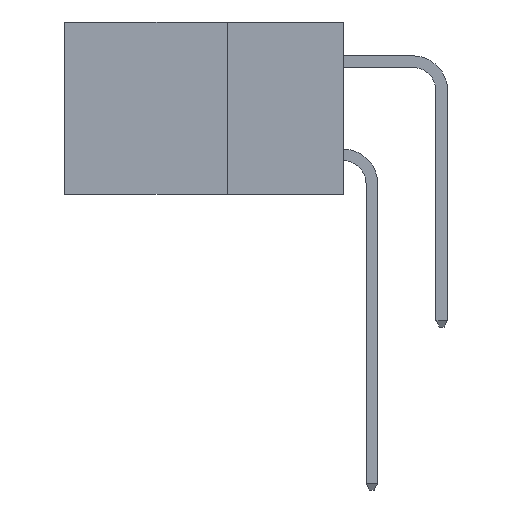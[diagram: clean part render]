
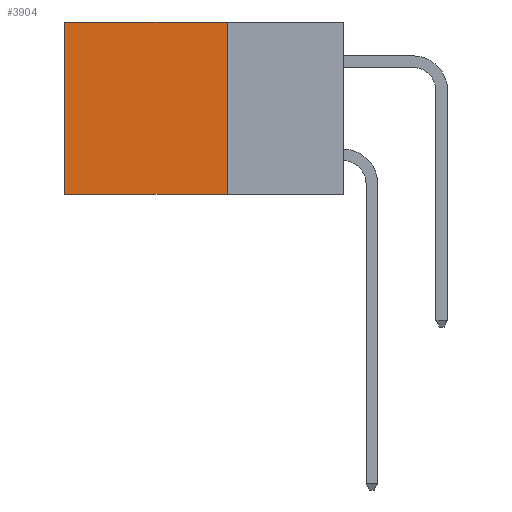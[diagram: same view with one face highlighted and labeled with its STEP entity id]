
A CAD part, left-side view. The second image highlights one B-rep face of the part: STEP entity #3904.
In plain terms, the highlighted planar face has unit normal (-1, 0, 0).
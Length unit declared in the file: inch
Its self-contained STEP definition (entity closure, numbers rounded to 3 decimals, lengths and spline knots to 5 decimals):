
#507 = CARTESIAN_POINT ( 'NONE',  ( 0.2615, 0.25, -0.37 ) ) ;
#1049 = CARTESIAN_POINT ( 'NONE',  ( 0.2615, 0.6, -0.37 ) ) ;
#1369 = ORIENTED_EDGE ( 'NONE', *, *, #10842, .F. ) ;
#2096 = CARTESIAN_POINT ( 'NONE',  ( 0.2615, 0.6, 0. ) ) ;
#2366 = AXIS2_PLACEMENT_3D ( 'NONE', #507, #11757, #5327 ) ;
#2974 = VERTEX_POINT ( 'NONE', #4627 ) ;
#3080 = EDGE_CURVE ( 'NONE', #2974, #10772, #5931, .T. ) ;
#3630 = CARTESIAN_POINT ( 'NONE',  ( 0.2615, 0.25, -0.37 ) ) ;
#3763 = ORIENTED_EDGE ( 'NONE', *, *, #10025, .T. ) ;
#3904 = ADVANCED_FACE ( 'NONE', ( #4700 ), #4205, .F. ) ;
#4205 = PLANE ( 'NONE',  #2366 ) ;
#4627 = CARTESIAN_POINT ( 'NONE',  ( 0.2615, 0.25, -0.37 ) ) ;
#4700 = FACE_OUTER_BOUND ( 'NONE', #9894, .T. ) ;
#5047 = CARTESIAN_POINT ( 'NONE',  ( 0.2615, 0.25, 0. ) ) ;
#5327 = DIRECTION ( 'NONE',  ( 0., 0., -1. ) ) ;
#5768 = VERTEX_POINT ( 'NONE', #5047 ) ;
#5931 = LINE ( 'NONE', #3630, #14060 ) ;
#5934 = LINE ( 'NONE', #9272, #14065 ) ;
#5939 = CARTESIAN_POINT ( 'NONE',  ( 0.2615, 0.6, -0.37 ) ) ;
#7885 = ORIENTED_EDGE ( 'NONE', *, *, #3080, .F. ) ;
#9147 = LINE ( 'NONE', #1049, #11979 ) ;
#9231 = VERTEX_POINT ( 'NONE', #2096 ) ;
#9272 = CARTESIAN_POINT ( 'NONE',  ( 0.2615, 0.25, -0.37 ) ) ;
#9894 = EDGE_LOOP ( 'NONE', ( #10147, #7885, #1369, #3763 ) ) ;
#9920 = EDGE_CURVE ( 'NONE', #9231, #10772, #9147, .T. ) ;
#10025 = EDGE_CURVE ( 'NONE', #5768, #9231, #11336, .T. ) ;
#10147 = ORIENTED_EDGE ( 'NONE', *, *, #9920, .T. ) ;
#10351 = DIRECTION ( 'NONE',  ( 0., 0., -1. ) ) ;
#10772 = VERTEX_POINT ( 'NONE', #5939 ) ;
#10842 = EDGE_CURVE ( 'NONE', #5768, #2974, #5934, .T. ) ;
#10936 = DIRECTION ( 'NONE',  ( 0., 0., -1. ) ) ;
#11336 = LINE ( 'NONE', #13222, #13460 ) ;
#11757 = DIRECTION ( 'NONE',  ( 1., 0., 0. ) ) ;
#11979 = VECTOR ( 'NONE', #10936, 39.37008 ) ;
#12173 = DIRECTION ( 'NONE',  ( 0., 1., 0. ) ) ;
#13222 = CARTESIAN_POINT ( 'NONE',  ( 0.2615, 0.25, 0. ) ) ;
#13287 = DIRECTION ( 'NONE',  ( 0., 1., 0. ) ) ;
#13460 = VECTOR ( 'NONE', #12173, 39.37008 ) ;
#14060 = VECTOR ( 'NONE', #13287, 39.37008 ) ;
#14065 = VECTOR ( 'NONE', #10351, 39.37008 ) ;
